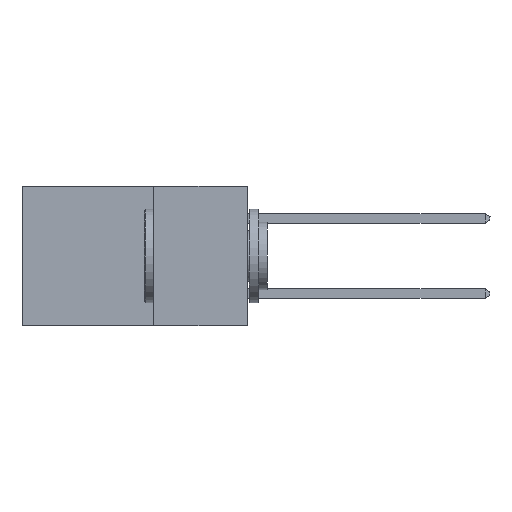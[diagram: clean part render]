
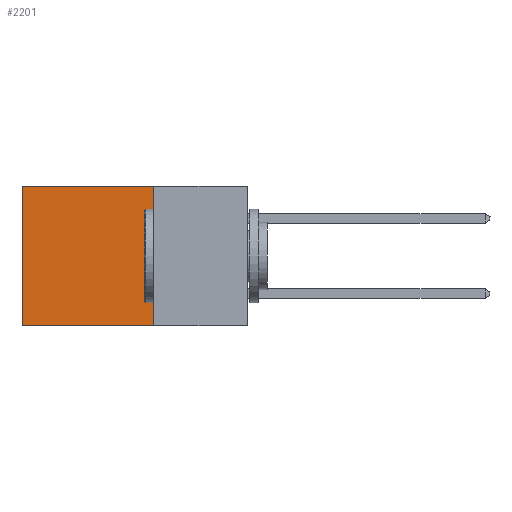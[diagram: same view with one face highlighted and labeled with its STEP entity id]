
A CAD part, left-side view. The second image highlights one B-rep face of the part: STEP entity #2201.
In plain terms, the highlighted planar face has unit normal (-1, 0, 0).
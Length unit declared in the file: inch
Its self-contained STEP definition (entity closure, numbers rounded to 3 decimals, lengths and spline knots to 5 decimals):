
#2 = VERTEX_POINT ( 'NONE', #7563 ) ;
#35 = DIRECTION ( 'NONE',  ( 0., 0., -1. ) ) ;
#101 = CARTESIAN_POINT ( 'NONE',  ( 0.298, 0.25, 0. ) ) ;
#115 = VECTOR ( 'NONE', #8327, 39.37008 ) ;
#583 = ORIENTED_EDGE ( 'NONE', *, *, #11877, .F. ) ;
#615 = VERTEX_POINT ( 'NONE', #4463 ) ;
#727 = CARTESIAN_POINT ( 'NONE',  ( 0.298, 0.25, 0. ) ) ;
#774 = PLANE ( 'NONE',  #9837 ) ;
#1054 = EDGE_CURVE ( 'NONE', #2, #9672, #4065, .T. ) ;
#2201 = ADVANCED_FACE ( 'NONE', ( #4338 ), #774, .F. ) ;
#2467 = CARTESIAN_POINT ( 'NONE',  ( 0.298, 0.6, -0.37 ) ) ;
#2934 = EDGE_CURVE ( 'NONE', #615, #2, #5989, .T. ) ;
#3866 = VECTOR ( 'NONE', #10782, 39.37008 ) ;
#4026 = ORIENTED_EDGE ( 'NONE', *, *, #2934, .T. ) ;
#4065 = LINE ( 'NONE', #9288, #115 ) ;
#4224 = EDGE_CURVE ( 'NONE', #615, #10653, #6983, .T. ) ;
#4338 = FACE_OUTER_BOUND ( 'NONE', #12516, .T. ) ;
#4425 = VECTOR ( 'NONE', #35, 39.37008 ) ;
#4463 = CARTESIAN_POINT ( 'NONE',  ( 0.298, 0.25, 0. ) ) ;
#5029 = VECTOR ( 'NONE', #10501, 39.37008 ) ;
#5852 = CARTESIAN_POINT ( 'NONE',  ( 0.298, 0.25, 0. ) ) ;
#5989 = LINE ( 'NONE', #101, #3866 ) ;
#6590 = CARTESIAN_POINT ( 'NONE',  ( 0.298, 0.25, -0.37 ) ) ;
#6983 = LINE ( 'NONE', #5852, #4425 ) ;
#7563 = CARTESIAN_POINT ( 'NONE',  ( 0.298, 0.6, 0. ) ) ;
#8327 = DIRECTION ( 'NONE',  ( 0., 0., -1. ) ) ;
#9288 = CARTESIAN_POINT ( 'NONE',  ( 0.298, 0.6, 0. ) ) ;
#9672 = VERTEX_POINT ( 'NONE', #2467 ) ;
#9837 = AXIS2_PLACEMENT_3D ( 'NONE', #727, #11442, #10560 ) ;
#10417 = CARTESIAN_POINT ( 'NONE',  ( 0.298, 0.25, -0.37 ) ) ;
#10501 = DIRECTION ( 'NONE',  ( 0., 1., 0. ) ) ;
#10560 = DIRECTION ( 'NONE',  ( 0., 0., -1. ) ) ;
#10653 = VERTEX_POINT ( 'NONE', #10417 ) ;
#10782 = DIRECTION ( 'NONE',  ( 0., 1., 0. ) ) ;
#10919 = LINE ( 'NONE', #6590, #5029 ) ;
#11089 = ORIENTED_EDGE ( 'NONE', *, *, #1054, .T. ) ;
#11414 = ORIENTED_EDGE ( 'NONE', *, *, #4224, .F. ) ;
#11442 = DIRECTION ( 'NONE',  ( 1., 0., 0. ) ) ;
#11877 = EDGE_CURVE ( 'NONE', #10653, #9672, #10919, .T. ) ;
#12516 = EDGE_LOOP ( 'NONE', ( #11089, #583, #11414, #4026 ) ) ;
